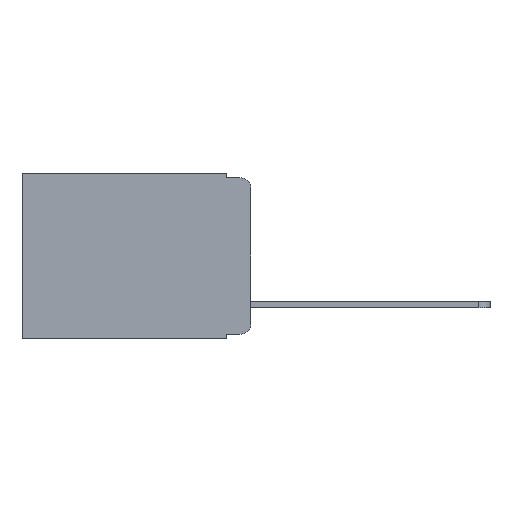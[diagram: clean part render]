
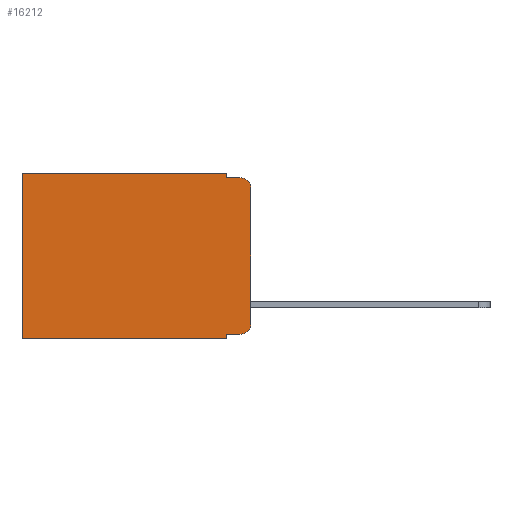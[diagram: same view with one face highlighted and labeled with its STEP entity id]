
A CAD part, left-side view. The second image highlights one B-rep face of the part: STEP entity #16212.
In plain terms, the highlighted planar face has unit normal (-1, 0, 0).
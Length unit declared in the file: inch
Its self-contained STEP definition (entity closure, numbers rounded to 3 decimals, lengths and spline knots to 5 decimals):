
#16 = ORIENTED_EDGE ( 'NONE', *, *, #15260, .T. ) ;
#56 = VERTEX_POINT ( 'NONE', #2750 ) ;
#1081 = AXIS2_PLACEMENT_3D ( 'NONE', #4147, #15042, #5666 ) ;
#1608 = EDGE_CURVE ( 'NONE', #56, #4926, #19632, .T. ) ;
#1733 = DIRECTION ( 'NONE',  ( 0., -1., 0. ) ) ;
#2002 = EDGE_CURVE ( 'NONE', #4926, #3286, #2259, .T. ) ;
#2259 = LINE ( 'NONE', #9613, #12279 ) ;
#2454 = DIRECTION ( 'NONE',  ( 0., 1., 0. ) ) ;
#2596 = VERTEX_POINT ( 'NONE', #13727 ) ;
#2750 = CARTESIAN_POINT ( 'NONE',  ( 0.298, 0.051, 0. ) ) ;
#2827 = CARTESIAN_POINT ( 'NONE',  ( 0.298, 0.02, -0.03 ) ) ;
#3286 = VERTEX_POINT ( 'NONE', #7619 ) ;
#4042 = ORIENTED_EDGE ( 'NONE', *, *, #2002, .F. ) ;
#4147 = CARTESIAN_POINT ( 'NONE',  ( 0.298, 0.02, -0.313 ) ) ;
#4158 = CARTESIAN_POINT ( 'NONE',  ( 0.298, 0., -0.03 ) ) ;
#4500 = CARTESIAN_POINT ( 'NONE',  ( 0.298, 0.051, -0.343 ) ) ;
#4787 = ORIENTED_EDGE ( 'NONE', *, *, #11817, .F. ) ;
#4898 = EDGE_CURVE ( 'NONE', #14006, #19402, #15581, .T. ) ;
#4926 = VERTEX_POINT ( 'NONE', #14617 ) ;
#5120 = LINE ( 'NONE', #14855, #6343 ) ;
#5666 = DIRECTION ( 'NONE',  ( 0., 0., -1. ) ) ;
#5876 = VERTEX_POINT ( 'NONE', #8146 ) ;
#6343 = VECTOR ( 'NONE', #6877, 39.37008 ) ;
#6665 = ORIENTED_EDGE ( 'NONE', *, *, #19771, .T. ) ;
#6877 = DIRECTION ( 'NONE',  ( 0., 0., -1. ) ) ;
#6909 = DIRECTION ( 'NONE',  ( 0., 0., -1. ) ) ;
#7240 = ORIENTED_EDGE ( 'NONE', *, *, #4898, .F. ) ;
#7312 = ORIENTED_EDGE ( 'NONE', *, *, #13613, .F. ) ;
#7619 = CARTESIAN_POINT ( 'NONE',  ( 0.298, 0.02, -0.01 ) ) ;
#7680 = CARTESIAN_POINT ( 'NONE',  ( 0.298, 0., 0. ) ) ;
#7790 = CARTESIAN_POINT ( 'NONE',  ( 0.298, 0.051, -0.333 ) ) ;
#7940 = DIRECTION ( 'NONE',  ( 0., 1., 0. ) ) ;
#8146 = CARTESIAN_POINT ( 'NONE',  ( 0.298, 0.473, -0.343 ) ) ;
#8500 = FACE_OUTER_BOUND ( 'NONE', #13455, .T. ) ;
#8504 = VECTOR ( 'NONE', #6909, 39.37008 ) ;
#8771 = CARTESIAN_POINT ( 'NONE',  ( 0.298, 0., -0.343 ) ) ;
#8892 = ORIENTED_EDGE ( 'NONE', *, *, #12670, .T. ) ;
#9009 = CARTESIAN_POINT ( 'NONE',  ( 0.298, 0.02, -0.333 ) ) ;
#9267 = LINE ( 'NONE', #7680, #15592 ) ;
#9613 = CARTESIAN_POINT ( 'NONE',  ( 0.298, 0.051, -0.01 ) ) ;
#10306 = VERTEX_POINT ( 'NONE', #9009 ) ;
#10740 = VECTOR ( 'NONE', #15621, 39.37008 ) ;
#11639 = CARTESIAN_POINT ( 'NONE',  ( 0.298, 0.051, 0. ) ) ;
#11817 = EDGE_CURVE ( 'NONE', #19330, #17043, #5120, .T. ) ;
#12173 = CARTESIAN_POINT ( 'NONE',  ( 0.298, 0.051, -0.333 ) ) ;
#12176 = LINE ( 'NONE', #7790, #18534 ) ;
#12279 = VECTOR ( 'NONE', #1733, 39.37008 ) ;
#12670 = EDGE_CURVE ( 'NONE', #56, #2596, #9267, .T. ) ;
#12976 = EDGE_CURVE ( 'NONE', #10306, #17043, #14129, .T. ) ;
#13296 = VECTOR ( 'NONE', #17606, 39.37008 ) ;
#13377 = VECTOR ( 'NONE', #2454, 39.37008 ) ;
#13455 = EDGE_LOOP ( 'NONE', ( #4787, #16317, #4042, #18031, #8892, #16, #7312, #7240, #6665, #16716 ) ) ;
#13613 = EDGE_CURVE ( 'NONE', #19402, #5876, #19720, .T. ) ;
#13727 = CARTESIAN_POINT ( 'NONE',  ( 0.298, 0.473, 0. ) ) ;
#14006 = VERTEX_POINT ( 'NONE', #12173 ) ;
#14129 = CIRCLE ( 'NONE', #1081, 0.02 ) ;
#14492 = AXIS2_PLACEMENT_3D ( 'NONE', #2827, #15633, #18917 ) ;
#14520 = CARTESIAN_POINT ( 'NONE',  ( 0.298, 0.051, 0. ) ) ;
#14617 = CARTESIAN_POINT ( 'NONE',  ( 0.298, 0.051, -0.01 ) ) ;
#14855 = CARTESIAN_POINT ( 'NONE',  ( 0.298, 0., 0. ) ) ;
#15042 = DIRECTION ( 'NONE',  ( -1., 0., 0. ) ) ;
#15260 = EDGE_CURVE ( 'NONE', #2596, #5876, #17817, .T. ) ;
#15402 = AXIS2_PLACEMENT_3D ( 'NONE', #20157, #18646, #18436 ) ;
#15581 = LINE ( 'NONE', #11639, #8504 ) ;
#15592 = VECTOR ( 'NONE', #7940, 39.37008 ) ;
#15621 = DIRECTION ( 'NONE',  ( 0., 0., -1. ) ) ;
#15633 = DIRECTION ( 'NONE',  ( -1., 0., 0. ) ) ;
#16212 = ADVANCED_FACE ( 'NONE', ( #8500 ), #20034, .F. ) ;
#16317 = ORIENTED_EDGE ( 'NONE', *, *, #17694, .T. ) ;
#16716 = ORIENTED_EDGE ( 'NONE', *, *, #12976, .T. ) ;
#16760 = CARTESIAN_POINT ( 'NONE',  ( 0.298, 0., -0.313 ) ) ;
#16975 = CARTESIAN_POINT ( 'NONE',  ( 0.298, 0.473, 0. ) ) ;
#17043 = VERTEX_POINT ( 'NONE', #16760 ) ;
#17606 = DIRECTION ( 'NONE',  ( 0., 0., -1. ) ) ;
#17694 = EDGE_CURVE ( 'NONE', #19330, #3286, #19654, .T. ) ;
#17817 = LINE ( 'NONE', #16975, #10740 ) ;
#18031 = ORIENTED_EDGE ( 'NONE', *, *, #1608, .F. ) ;
#18436 = DIRECTION ( 'NONE',  ( 0., 0., -1. ) ) ;
#18534 = VECTOR ( 'NONE', #18792, 39.37008 ) ;
#18646 = DIRECTION ( 'NONE',  ( 1., 0., 0. ) ) ;
#18792 = DIRECTION ( 'NONE',  ( 0., -1., 0. ) ) ;
#18917 = DIRECTION ( 'NONE',  ( 0., 0., -1. ) ) ;
#19330 = VERTEX_POINT ( 'NONE', #4158 ) ;
#19402 = VERTEX_POINT ( 'NONE', #4500 ) ;
#19632 = LINE ( 'NONE', #14520, #13296 ) ;
#19654 = CIRCLE ( 'NONE', #14492, 0.02 ) ;
#19720 = LINE ( 'NONE', #8771, #13377 ) ;
#19771 = EDGE_CURVE ( 'NONE', #14006, #10306, #12176, .T. ) ;
#20034 = PLANE ( 'NONE',  #15402 ) ;
#20157 = CARTESIAN_POINT ( 'NONE',  ( 0.298, 0., 0. ) ) ;
